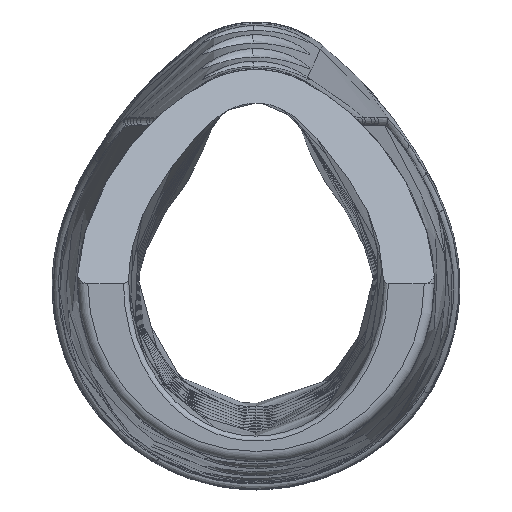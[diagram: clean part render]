
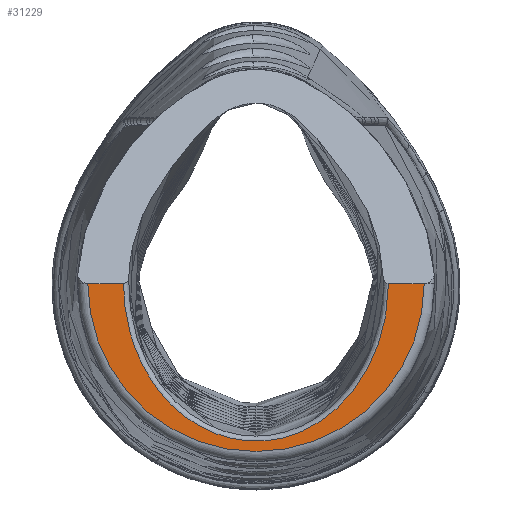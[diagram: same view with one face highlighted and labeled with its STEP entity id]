
A CAD part, top view. The second image highlights one B-rep face of the part: STEP entity #31229.
In plain terms, the highlighted planar face has unit normal (0, 0, 1).
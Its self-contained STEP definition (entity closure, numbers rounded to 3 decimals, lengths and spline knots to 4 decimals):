
#985 = EDGE_CURVE ( 'NONE', #6447, #14746, #5879, .T. ) ;
#1717 = EDGE_CURVE ( 'NONE', #29297, #29997, #11247, .T. ) ;
#2128 = DIRECTION ( 'NONE',  ( -1., 0., 0. ) ) ;
#2204 = DIRECTION ( 'NONE',  ( -1., 0., 0. ) ) ;
#2645 = CARTESIAN_POINT ( 'NONE',  ( 0.4496, -0.5616, 8.25 ) ) ;
#2842 = CARTESIAN_POINT ( 'NONE',  ( -0.0957, -0.7665, 8.25 ) ) ;
#3035 = CARTESIAN_POINT ( 'NONE',  ( 0.531, -0.4472, 8.25 ) ) ;
#3414 = CARTESIAN_POINT ( 'NONE',  ( -0.2289, -0.7269, 8.25 ) ) ;
#3879 = CARTESIAN_POINT ( 'NONE',  ( -0.825, -0.0014, 8.25 ) ) ;
#5550 = CARTESIAN_POINT ( 'NONE',  ( -0.4509, -0.5584, 8.25 ) ) ;
#5879 = LINE ( 'NONE', #32302, #29595 ) ;
#5926 = CARTESIAN_POINT ( 'NONE',  ( 0.4177, -0.5957, 8.25 ) ) ;
#6112 = CARTESIAN_POINT ( 'NONE',  ( -0.6461, -0.0947, 8.25 ) ) ;
#6296 = CARTESIAN_POINT ( 'NONE',  ( 0.506, -0.4866, 8.25 ) ) ;
#6447 = VERTEX_POINT ( 'NONE', #36741 ) ;
#8293 = CIRCLE ( 'NONE', #29848, 0.825 ) ;
#8437 = CARTESIAN_POINT ( 'NONE',  ( 0.3076, -0.6828, 8.25 ) ) ;
#8499 = PLANE ( 'NONE',  #35861 ) ;
#8512 = ORIENTED_EDGE ( 'NONE', *, *, #1717, .T. ) ;
#8631 = CARTESIAN_POINT ( 'NONE',  ( 0.3461, -0.6561, 8.25 ) ) ;
#9005 = CARTESIAN_POINT ( 'NONE',  ( 0.6489, -0.0483, 8.25 ) ) ;
#9190 = CARTESIAN_POINT ( 'NONE',  ( 0.4926, -0.5059, 8.25 ) ) ;
#10575 = EDGE_CURVE ( 'NONE', #29997, #6447, #17985, .T. ) ;
#11247 = LINE ( 'NONE', #28623, #23427 ) ;
#11314 = CARTESIAN_POINT ( 'NONE',  ( 0.1817, -0.7438, 8.25 ) ) ;
#11376 = DIRECTION ( 'NONE',  ( 0., 0., -1. ) ) ;
#11511 = CARTESIAN_POINT ( 'NONE',  ( -0.4661, -0.5404, 8.25 ) ) ;
#11890 = CARTESIAN_POINT ( 'NONE',  ( -0.049, -0.7728, 8.25 ) ) ;
#12075 = CARTESIAN_POINT ( 'NONE',  ( -0.5743, -0.3633, 8.25 ) ) ;
#13869 = CARTESIAN_POINT ( 'NONE',  ( 0.825, -0.0014, 8.25 ) ) ;
#14244 = ORIENTED_EDGE ( 'NONE', *, *, #10575, .T. ) ;
#14393 = CARTESIAN_POINT ( 'NONE',  ( -0.6498, -0.0483, 8.25 ) ) ;
#14592 = CARTESIAN_POINT ( 'NONE',  ( -0.4189, -0.5927, 8.25 ) ) ;
#14746 = VERTEX_POINT ( 'NONE', #3879 ) ;
#14780 = CARTESIAN_POINT ( 'NONE',  ( -0.3108, -0.6807, 8.25 ) ) ;
#14965 = CARTESIAN_POINT ( 'NONE',  ( 0.5917, -0.3213, 8.25 ) ) ;
#16783 = DIRECTION ( 'NONE',  ( 0., 0., 1. ) ) ;
#17302 = CARTESIAN_POINT ( 'NONE',  ( -0.5084, -0.4851, 8.25 ) ) ;
#17494 = CARTESIAN_POINT ( 'NONE',  ( 0.0453, -0.7746, 8.25 ) ) ;
#17682 = CARTESIAN_POINT ( 'NONE',  ( 0.6452, -0.0949, 8.25 ) ) ;
#17985 = B_SPLINE_CURVE_WITH_KNOTS ( 'NONE', 3,
 ( #33919, #20758, #9005, #17682, #29453, #37772, #23273, #20940, #14965, #35061, #32729, #23466, #3035, #6296, #9190, #2645, #5926, #23077, #8631, #8437, #18055, #29259, #20569, #23839, #11314, #26738, #29826, #35625, #17494, #20381, #11890, #2842, #25976, #26354, #3414, #31971, #14780, #20189, #35252, #34865, #14592, #5550, #11511, #17302, #26166, #32164, #12075, #35441, #29639, #26546, #29063, #6112, #14393, #32353 ),
 .UNSPECIFIED., .F., .F.,
 ( 4, 2, 2, 2, 2, 2, 2, 2, 2, 2, 2, 2, 2, 2, 2, 2, 2, 2, 2, 2, 2, 2, 2, 2, 2, 2, 4 ),
 ( 0.0309, 0.0327, 0.0345, 0.0381, 0.0399, 0.0417, 0.0435, 0.0453, 0.0489, 0.0507, 0.0525, 0.0543, 0.0552, 0.0561, 0.0597, 0.0615, 0.0633, 0.067, 0.0688, 0.0706, 0.0724, 0.0742, 0.0778, 0.0796, 0.0814, 0.085, 0.0886 ),
 .UNSPECIFIED. ) ;
#18055 = CARTESIAN_POINT ( 'NONE',  ( 0.2877, -0.695, 8.25 ) ) ;
#19670 = CARTESIAN_POINT ( 'NONE',  ( 0., 0., 8.25 ) ) ;
#20189 = CARTESIAN_POINT ( 'NONE',  ( -0.3489, -0.654, 8.25 ) ) ;
#20252 = DIRECTION ( 'NONE',  ( -1., 0., 0. ) ) ;
#20361 = ORIENTED_EDGE ( 'NONE', *, *, #25458, .T. ) ;
#20381 = CARTESIAN_POINT ( 'NONE',  ( -0.0255, -0.7744, 8.25 ) ) ;
#20569 = CARTESIAN_POINT ( 'NONE',  ( 0.2255, -0.7269, 8.25 ) ) ;
#20758 = CARTESIAN_POINT ( 'NONE',  ( 0.6498, -0.0248, 8.25 ) ) ;
#20816 = CARTESIAN_POINT ( 'NONE',  ( 0., 0., 8.25 ) ) ;
#20940 = CARTESIAN_POINT ( 'NONE',  ( 0.5998, -0.2991, 8.25 ) ) ;
#21297 = CARTESIAN_POINT ( 'NONE',  ( 0.6498, -0.0014, 8.25 ) ) ;
#22962 = ORIENTED_EDGE ( 'NONE', *, *, #985, .T. ) ;
#23077 = CARTESIAN_POINT ( 'NONE',  ( 0.3648, -0.6416, 8.25 ) ) ;
#23273 = CARTESIAN_POINT ( 'NONE',  ( 0.6212, -0.2323, 8.25 ) ) ;
#23427 = VECTOR ( 'NONE', #2204, 39.3701 ) ;
#23466 = CARTESIAN_POINT ( 'NONE',  ( 0.5426, -0.427, 8.25 ) ) ;
#23839 = CARTESIAN_POINT ( 'NONE',  ( 0.1928, -0.7398, 8.25 ) ) ;
#25458 = EDGE_CURVE ( 'NONE', #14746, #29297, #8293, .T. ) ;
#25976 = CARTESIAN_POINT ( 'NONE',  ( -0.1186, -0.762, 8.25 ) ) ;
#26166 = CARTESIAN_POINT ( 'NONE',  ( -0.5329, -0.4459, 8.25 ) ) ;
#26354 = CARTESIAN_POINT ( 'NONE',  ( -0.1858, -0.7442, 8.25 ) ) ;
#26546 = CARTESIAN_POINT ( 'NONE',  ( -0.6215, -0.2313, 8.25 ) ) ;
#26738 = CARTESIAN_POINT ( 'NONE',  ( 0.1593, -0.751, 8.25 ) ) ;
#28623 = CARTESIAN_POINT ( 'NONE',  ( 0., -0.0014, 8.25 ) ) ;
#29063 = CARTESIAN_POINT ( 'NONE',  ( -0.632, -0.1862, 8.25 ) ) ;
#29259 = CARTESIAN_POINT ( 'NONE',  ( 0.2467, -0.7171, 8.25 ) ) ;
#29297 = VERTEX_POINT ( 'NONE', #13869 ) ;
#29405 = DIRECTION ( 'NONE',  ( -1., 0., 0. ) ) ;
#29453 = CARTESIAN_POINT ( 'NONE',  ( 0.6425, -0.1181, 8.25 ) ) ;
#29595 = VECTOR ( 'NONE', #29405, 39.3701 ) ;
#29639 = CARTESIAN_POINT ( 'NONE',  ( -0.6002, -0.298, 8.25 ) ) ;
#29826 = CARTESIAN_POINT ( 'NONE',  ( 0.148, -0.7542, 8.25 ) ) ;
#29848 = AXIS2_PLACEMENT_3D ( 'NONE', #19670, #16783, #2128 ) ;
#29997 = VERTEX_POINT ( 'NONE', #21297 ) ;
#30653 = EDGE_LOOP ( 'NONE', ( #20361, #8512, #14244, #22962 ) ) ;
#31229 = ADVANCED_FACE ( 'NONE', ( #35499 ), #8499, .F. ) ;
#31971 = CARTESIAN_POINT ( 'NONE',  ( -0.2909, -0.6931, 8.25 ) ) ;
#32164 = CARTESIAN_POINT ( 'NONE',  ( -0.5646, -0.3843, 8.25 ) ) ;
#32302 = CARTESIAN_POINT ( 'NONE',  ( 0., -0.0014, 8.25 ) ) ;
#32353 = CARTESIAN_POINT ( 'NONE',  ( -0.6498, -0.0014, 8.25 ) ) ;
#32729 = CARTESIAN_POINT ( 'NONE',  ( 0.564, -0.3856, 8.25 ) ) ;
#33919 = CARTESIAN_POINT ( 'NONE',  ( 0.6498, -0.0014, 8.25 ) ) ;
#34865 = CARTESIAN_POINT ( 'NONE',  ( -0.4022, -0.609, 8.25 ) ) ;
#35061 = CARTESIAN_POINT ( 'NONE',  ( 0.5738, -0.3645, 8.25 ) ) ;
#35252 = CARTESIAN_POINT ( 'NONE',  ( -0.3672, -0.6396, 8.25 ) ) ;
#35441 = CARTESIAN_POINT ( 'NONE',  ( -0.5921, -0.3202, 8.25 ) ) ;
#35499 = FACE_OUTER_BOUND ( 'NONE', #30653, .T. ) ;
#35625 = CARTESIAN_POINT ( 'NONE',  ( 0.0915, -0.7687, 8.25 ) ) ;
#35861 = AXIS2_PLACEMENT_3D ( 'NONE', #20816, #11376, #20252 ) ;
#36741 = CARTESIAN_POINT ( 'NONE',  ( -0.6498, -0.0014, 8.25 ) ) ;
#37772 = CARTESIAN_POINT ( 'NONE',  ( 0.6318, -0.187, 8.25 ) ) ;
